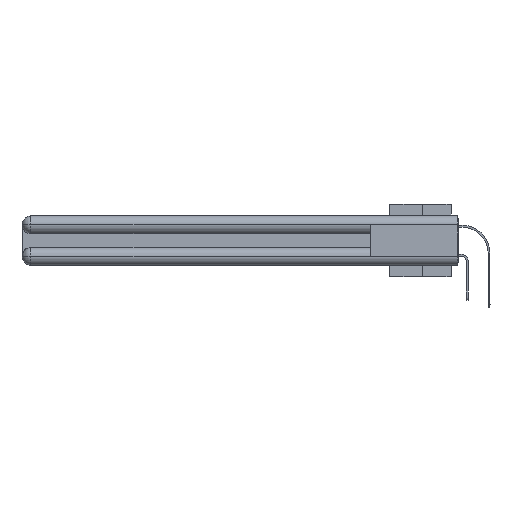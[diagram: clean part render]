
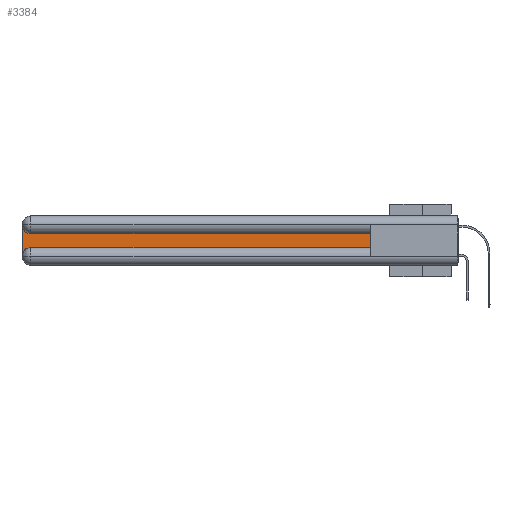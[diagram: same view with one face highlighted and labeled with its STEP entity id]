
A CAD part, left-side view. The second image highlights one B-rep face of the part: STEP entity #3384.
In plain terms, the highlighted planar face has unit normal (-1, 0, 0).
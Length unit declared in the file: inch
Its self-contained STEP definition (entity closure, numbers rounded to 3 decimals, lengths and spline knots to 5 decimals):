
#2029 = VERTEX_POINT ( 'NONE', #20035 ) ;
#2600 = DIRECTION ( 'NONE',  ( 1., 0., 0. ) ) ;
#3197 = CIRCLE ( 'NONE', #33785, 0.06 ) ;
#3384 = ADVANCED_FACE ( 'NONE', ( #13205 ), #18343, .F. ) ;
#3785 = EDGE_CURVE ( 'NONE', #14249, #31630, #23748, .T. ) ;
#4469 = DIRECTION ( 'NONE',  ( 1., 0., 0. ) ) ;
#5113 = EDGE_CURVE ( 'NONE', #9305, #2029, #17916, .T. ) ;
#5780 = ORIENTED_EDGE ( 'NONE', *, *, #5113, .T. ) ;
#5805 = DIRECTION ( 'NONE',  ( 0., 0., -1. ) ) ;
#6580 = EDGE_LOOP ( 'NONE', ( #5780, #19321, #26290, #6989, #32480, #27329 ) ) ;
#6620 = LINE ( 'NONE', #25115, #29674 ) ;
#6718 = EDGE_CURVE ( 'NONE', #25732, #30070, #29570, .T. ) ;
#6793 = DIRECTION ( 'NONE',  ( 0., 0., 1. ) ) ;
#6808 = EDGE_CURVE ( 'NONE', #31630, #9305, #6620, .T. ) ;
#6985 = AXIS2_PLACEMENT_3D ( 'NONE', #7544, #2600, #25707 ) ;
#6989 = ORIENTED_EDGE ( 'NONE', *, *, #22030, .T. ) ;
#7544 = CARTESIAN_POINT ( 'NONE',  ( 0.075, 3., -0.1225 ) ) ;
#8317 = CARTESIAN_POINT ( 'NONE',  ( 0.075, 0.6, -0.2175 ) ) ;
#8349 = CARTESIAN_POINT ( 'NONE',  ( 0.075, 3., -0.2175 ) ) ;
#8685 = DIRECTION ( 'NONE',  ( 0., 0., -1. ) ) ;
#9305 = VERTEX_POINT ( 'NONE', #27596 ) ;
#12768 = DIRECTION ( 'NONE',  ( 0., 1., 0. ) ) ;
#13205 = FACE_OUTER_BOUND ( 'NONE', #6580, .T. ) ;
#14249 = VERTEX_POINT ( 'NONE', #15298 ) ;
#15298 = CARTESIAN_POINT ( 'NONE',  ( 0.075, 2.94, -0.2175 ) ) ;
#17916 = LINE ( 'NONE', #20311, #31940 ) ;
#18343 = PLANE ( 'NONE',  #6985 ) ;
#18827 = AXIS2_PLACEMENT_3D ( 'NONE', #22959, #4469, #25678 ) ;
#19311 = DIRECTION ( 'NONE',  ( 1., 0., 0. ) ) ;
#19321 = ORIENTED_EDGE ( 'NONE', *, *, #25250, .T. ) ;
#20035 = CARTESIAN_POINT ( 'NONE',  ( 0.075, 2.94, -0.1225 ) ) ;
#20311 = CARTESIAN_POINT ( 'NONE',  ( 0.075, 0.6, -0.1225 ) ) ;
#22030 = EDGE_CURVE ( 'NONE', #30070, #14249, #33546, .T. ) ;
#22959 = CARTESIAN_POINT ( 'NONE',  ( 0.075, 2.94, -0.2775 ) ) ;
#23748 = LINE ( 'NONE', #8317, #29715 ) ;
#25115 = CARTESIAN_POINT ( 'NONE',  ( 0.075, 0.6, -0.2175 ) ) ;
#25250 = EDGE_CURVE ( 'NONE', #2029, #25732, #3197, .T. ) ;
#25291 = VECTOR ( 'NONE', #5805, 39.37008 ) ;
#25298 = CARTESIAN_POINT ( 'NONE',  ( 0.075, 3., -0.2775 ) ) ;
#25678 = DIRECTION ( 'NONE',  ( 0., 0., -1. ) ) ;
#25707 = DIRECTION ( 'NONE',  ( 0., 0., -1. ) ) ;
#25732 = VERTEX_POINT ( 'NONE', #26550 ) ;
#26290 = ORIENTED_EDGE ( 'NONE', *, *, #6718, .T. ) ;
#26550 = CARTESIAN_POINT ( 'NONE',  ( 0.075, 3., -0.0625 ) ) ;
#27329 = ORIENTED_EDGE ( 'NONE', *, *, #6808, .T. ) ;
#27596 = CARTESIAN_POINT ( 'NONE',  ( 0.075, 0.6, -0.1225 ) ) ;
#28857 = DIRECTION ( 'NONE',  ( 0., -1., 0. ) ) ;
#29094 = CARTESIAN_POINT ( 'NONE',  ( 0.075, 0.6, -0.2175 ) ) ;
#29570 = LINE ( 'NONE', #8349, #25291 ) ;
#29674 = VECTOR ( 'NONE', #6793, 39.37008 ) ;
#29715 = VECTOR ( 'NONE', #28857, 39.37008 ) ;
#30070 = VERTEX_POINT ( 'NONE', #25298 ) ;
#31630 = VERTEX_POINT ( 'NONE', #29094 ) ;
#31940 = VECTOR ( 'NONE', #12768, 39.37008 ) ;
#32144 = CARTESIAN_POINT ( 'NONE',  ( 0.075, 2.94, -0.0625 ) ) ;
#32480 = ORIENTED_EDGE ( 'NONE', *, *, #3785, .T. ) ;
#33546 = CIRCLE ( 'NONE', #18827, 0.06 ) ;
#33785 = AXIS2_PLACEMENT_3D ( 'NONE', #32144, #19311, #8685 ) ;
